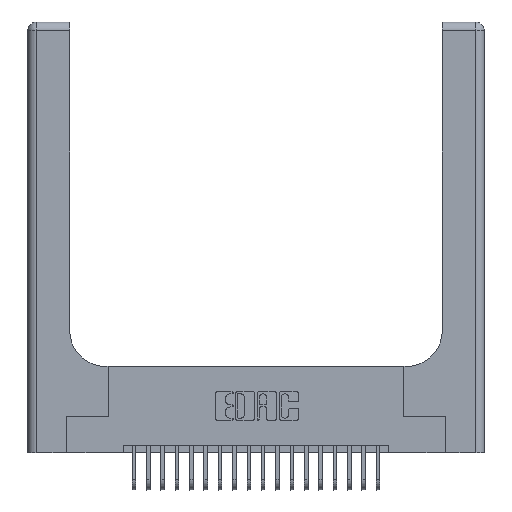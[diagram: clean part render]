
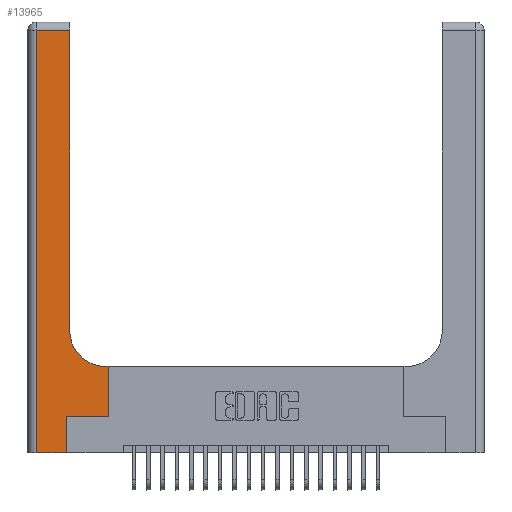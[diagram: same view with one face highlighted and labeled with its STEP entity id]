
A CAD part, top view. The second image highlights one B-rep face of the part: STEP entity #13965.
In plain terms, the highlighted planar face has unit normal (0, 0, 1).
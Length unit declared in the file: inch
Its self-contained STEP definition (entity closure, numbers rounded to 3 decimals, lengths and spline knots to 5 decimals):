
#527 = VERTEX_POINT ( 'NONE', #7596 ) ;
#1077 = LINE ( 'NONE', #18317, #15403 ) ;
#1162 = CARTESIAN_POINT ( 'NONE',  ( 0.2915, 0.85, 0.37 ) ) ;
#2027 = ORIENTED_EDGE ( 'NONE', *, *, #18040, .T. ) ;
#2129 = CARTESIAN_POINT ( 'NONE',  ( 0.5415, 0.6, 0.37 ) ) ;
#2281 = CARTESIAN_POINT ( 'NONE',  ( 0.2915, 2.94, 0.37 ) ) ;
#2616 = CARTESIAN_POINT ( 'NONE',  ( 0.5585, 0.25, 0.37 ) ) ;
#3267 = LINE ( 'NONE', #3352, #16093 ) ;
#3352 = CARTESIAN_POINT ( 'NONE',  ( 0., 0., 0.37 ) ) ;
#3451 = DIRECTION ( 'NONE',  ( 0., 0., -1. ) ) ;
#3727 = CARTESIAN_POINT ( 'NONE',  ( 0., 3., 0.37 ) ) ;
#3876 = VECTOR ( 'NONE', #14996, 39.37008 ) ;
#4002 = CARTESIAN_POINT ( 'NONE',  ( 0.06, 3., 0.37 ) ) ;
#4678 = ORIENTED_EDGE ( 'NONE', *, *, #20979, .T. ) ;
#4784 = CARTESIAN_POINT ( 'NONE',  ( 0.269, 0., 0.37 ) ) ;
#4881 = AXIS2_PLACEMENT_3D ( 'NONE', #11050, #3451, #22162 ) ;
#5623 = VECTOR ( 'NONE', #17790, 39.37008 ) ;
#5920 = LINE ( 'NONE', #4002, #3876 ) ;
#6099 = VECTOR ( 'NONE', #9424, 39.37008 ) ;
#6170 = ORIENTED_EDGE ( 'NONE', *, *, #7022, .T. ) ;
#6679 = LINE ( 'NONE', #16873, #6099 ) ;
#6757 = EDGE_CURVE ( 'NONE', #14986, #19548, #6679, .T. ) ;
#6969 = DIRECTION ( 'NONE',  ( -1., 0., 0. ) ) ;
#7022 = EDGE_CURVE ( 'NONE', #19548, #16065, #1077, .T. ) ;
#7382 = EDGE_CURVE ( 'NONE', #16065, #23676, #21259, .T. ) ;
#7471 = CARTESIAN_POINT ( 'NONE',  ( 0.269, 0., 0.37 ) ) ;
#7596 = CARTESIAN_POINT ( 'NONE',  ( 0.06, 0., 0.37 ) ) ;
#7634 = CARTESIAN_POINT ( 'NONE',  ( 0.06, 2.94, 0.37 ) ) ;
#7638 = DIRECTION ( 'NONE',  ( -1., 0., 0. ) ) ;
#7802 = DIRECTION ( 'NONE',  ( 0., 0., -1. ) ) ;
#9424 = DIRECTION ( 'NONE',  ( 1., 0., 0. ) ) ;
#10401 = EDGE_CURVE ( 'NONE', #16041, #14986, #17418, .T. ) ;
#10505 = ORIENTED_EDGE ( 'NONE', *, *, #16452, .T. ) ;
#10871 = DIRECTION ( 'NONE',  ( 1., 0., 0. ) ) ;
#11050 = CARTESIAN_POINT ( 'NONE',  ( 0.5415, 0.85, 0.37 ) ) ;
#11167 = PLANE ( 'NONE',  #23125 ) ;
#11175 = FACE_OUTER_BOUND ( 'NONE', #18175, .T. ) ;
#11338 = VECTOR ( 'NONE', #7638, 39.37008 ) ;
#12205 = VERTEX_POINT ( 'NONE', #1162 ) ;
#12559 = ORIENTED_EDGE ( 'NONE', *, *, #10401, .T. ) ;
#13529 = LINE ( 'NONE', #21412, #5623 ) ;
#13659 = CARTESIAN_POINT ( 'NONE',  ( 0.269, 0.25, 0.37 ) ) ;
#13965 = ADVANCED_FACE ( 'NONE', ( #11175 ), #11167, .F. ) ;
#14500 = VERTEX_POINT ( 'NONE', #7634 ) ;
#14634 = DIRECTION ( 'NONE',  ( 0., 1., 0. ) ) ;
#14917 = ORIENTED_EDGE ( 'NONE', *, *, #6757, .T. ) ;
#14986 = VERTEX_POINT ( 'NONE', #13659 ) ;
#14996 = DIRECTION ( 'NONE',  ( 0., -1., 0. ) ) ;
#15116 = VERTEX_POINT ( 'NONE', #2281 ) ;
#15403 = VECTOR ( 'NONE', #14634, 39.37008 ) ;
#15643 = CIRCLE ( 'NONE', #4881, 0.25 ) ;
#15979 = ORIENTED_EDGE ( 'NONE', *, *, #7382, .T. ) ;
#16041 = VERTEX_POINT ( 'NONE', #7471 ) ;
#16065 = VERTEX_POINT ( 'NONE', #18573 ) ;
#16093 = VECTOR ( 'NONE', #10871, 39.37008 ) ;
#16452 = EDGE_CURVE ( 'NONE', #527, #16041, #3267, .T. ) ;
#16602 = ORIENTED_EDGE ( 'NONE', *, *, #18439, .T. ) ;
#16873 = CARTESIAN_POINT ( 'NONE',  ( 0.269, 0.25, 0.37 ) ) ;
#17418 = LINE ( 'NONE', #4784, #18004 ) ;
#17790 = DIRECTION ( 'NONE',  ( 0., 1., 0. ) ) ;
#18004 = VECTOR ( 'NONE', #19584, 39.37008 ) ;
#18040 = EDGE_CURVE ( 'NONE', #12205, #15116, #13529, .T. ) ;
#18175 = EDGE_LOOP ( 'NONE', ( #2027, #4678, #16602, #10505, #12559, #14917, #6170, #15979, #19213 ) ) ;
#18317 = CARTESIAN_POINT ( 'NONE',  ( 0.5585, 0.25, 0.37 ) ) ;
#18439 = EDGE_CURVE ( 'NONE', #14500, #527, #5920, .T. ) ;
#18573 = CARTESIAN_POINT ( 'NONE',  ( 0.5585, 0.6, 0.37 ) ) ;
#18804 = CARTESIAN_POINT ( 'NONE',  ( 0.2915, 0.6, 0.37 ) ) ;
#19213 = ORIENTED_EDGE ( 'NONE', *, *, #22201, .T. ) ;
#19548 = VERTEX_POINT ( 'NONE', #2616 ) ;
#19584 = DIRECTION ( 'NONE',  ( 0., 1., 0. ) ) ;
#20979 = EDGE_CURVE ( 'NONE', #15116, #14500, #23896, .T. ) ;
#21259 = LINE ( 'NONE', #18804, #11338 ) ;
#21412 = CARTESIAN_POINT ( 'NONE',  ( 0.2915, 3., 0.37 ) ) ;
#22162 = DIRECTION ( 'NONE',  ( 1., 0., 0. ) ) ;
#22164 = CARTESIAN_POINT ( 'NONE',  ( 0., 2.94, 0.37 ) ) ;
#22201 = EDGE_CURVE ( 'NONE', #23676, #12205, #15643, .T. ) ;
#22451 = VECTOR ( 'NONE', #6969, 39.37008 ) ;
#22757 = DIRECTION ( 'NONE',  ( -1., 0., 0. ) ) ;
#23125 = AXIS2_PLACEMENT_3D ( 'NONE', #3727, #7802, #22757 ) ;
#23676 = VERTEX_POINT ( 'NONE', #2129 ) ;
#23896 = LINE ( 'NONE', #22164, #22451 ) ;
